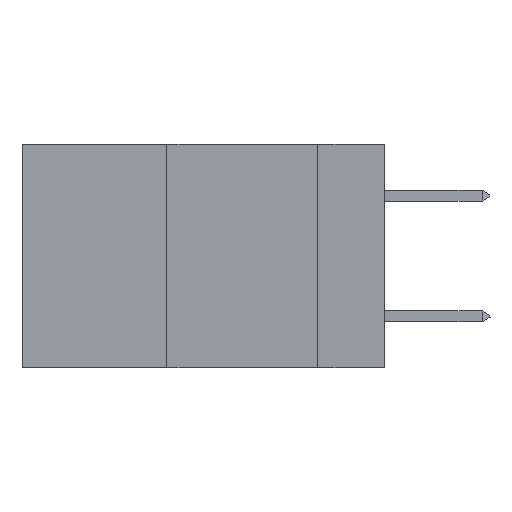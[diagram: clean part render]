
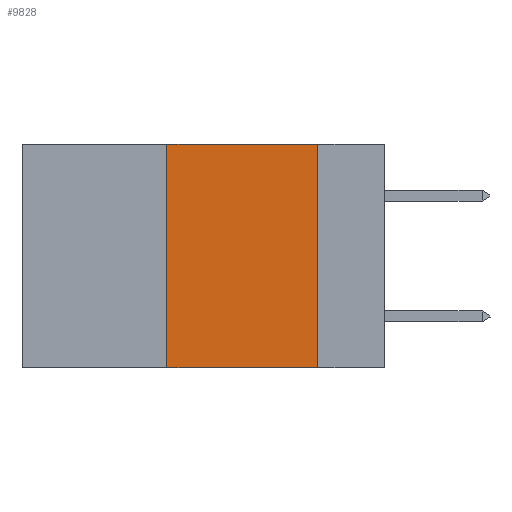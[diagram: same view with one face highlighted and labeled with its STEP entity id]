
A CAD part, left-side view. The second image highlights one B-rep face of the part: STEP entity #9828.
In plain terms, the highlighted planar face has unit normal (-1, 0, 0).
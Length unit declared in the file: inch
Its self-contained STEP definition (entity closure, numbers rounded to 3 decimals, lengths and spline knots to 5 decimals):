
#468 = CARTESIAN_POINT ( 'NONE',  ( 0., 0.36, -0.37 ) ) ;
#476 = AXIS2_PLACEMENT_3D ( 'NONE', #8048, #14608, #2676 ) ;
#2056 = DIRECTION ( 'NONE',  ( 0., -1., 0. ) ) ;
#2609 = EDGE_CURVE ( 'NONE', #14202, #14393, #5474, .T. ) ;
#2676 = DIRECTION ( 'NONE',  ( 0., 0., -1. ) ) ;
#3397 = EDGE_CURVE ( 'NONE', #8338, #14202, #6496, .T. ) ;
#3610 = EDGE_LOOP ( 'NONE', ( #13417, #13949, #13427, #10322 ) ) ;
#3823 = LINE ( 'NONE', #16042, #7679 ) ;
#4087 = EDGE_CURVE ( 'NONE', #5203, #8338, #3823, .T. ) ;
#4833 = EDGE_CURVE ( 'NONE', #5203, #14393, #5426, .T. ) ;
#5203 = VERTEX_POINT ( 'NONE', #468 ) ;
#5362 = CARTESIAN_POINT ( 'NONE',  ( 0., 0.11, -0.37 ) ) ;
#5426 = LINE ( 'NONE', #8426, #8472 ) ;
#5474 = LINE ( 'NONE', #16854, #6697 ) ;
#5639 = DIRECTION ( 'NONE',  ( 0., -1., 0. ) ) ;
#6496 = LINE ( 'NONE', #14691, #10922 ) ;
#6697 = VECTOR ( 'NONE', #7097, 39.37008 ) ;
#7097 = DIRECTION ( 'NONE',  ( 0., 0., -1. ) ) ;
#7679 = VECTOR ( 'NONE', #14783, 39.37008 ) ;
#8048 = CARTESIAN_POINT ( 'NONE',  ( 0., 0.6, 0. ) ) ;
#8338 = VERTEX_POINT ( 'NONE', #16804 ) ;
#8426 = CARTESIAN_POINT ( 'NONE',  ( 0., 0.6, -0.37 ) ) ;
#8472 = VECTOR ( 'NONE', #2056, 39.37008 ) ;
#9828 = ADVANCED_FACE ( 'NONE', ( #11784 ), #10613, .F. ) ;
#10322 = ORIENTED_EDGE ( 'NONE', *, *, #4833, .T. ) ;
#10613 = PLANE ( 'NONE',  #476 ) ;
#10922 = VECTOR ( 'NONE', #5639, 39.37008 ) ;
#11784 = FACE_OUTER_BOUND ( 'NONE', #3610, .T. ) ;
#12464 = CARTESIAN_POINT ( 'NONE',  ( 0., 0.11, 0. ) ) ;
#13417 = ORIENTED_EDGE ( 'NONE', *, *, #2609, .F. ) ;
#13427 = ORIENTED_EDGE ( 'NONE', *, *, #4087, .F. ) ;
#13949 = ORIENTED_EDGE ( 'NONE', *, *, #3397, .F. ) ;
#14202 = VERTEX_POINT ( 'NONE', #12464 ) ;
#14393 = VERTEX_POINT ( 'NONE', #5362 ) ;
#14608 = DIRECTION ( 'NONE',  ( 1., 0., 0. ) ) ;
#14691 = CARTESIAN_POINT ( 'NONE',  ( 0., 0.6, 0. ) ) ;
#14783 = DIRECTION ( 'NONE',  ( 0., 0., 1. ) ) ;
#16042 = CARTESIAN_POINT ( 'NONE',  ( 0., 0.36, 0. ) ) ;
#16804 = CARTESIAN_POINT ( 'NONE',  ( 0., 0.36, 0. ) ) ;
#16854 = CARTESIAN_POINT ( 'NONE',  ( 0., 0.11, 0. ) ) ;
